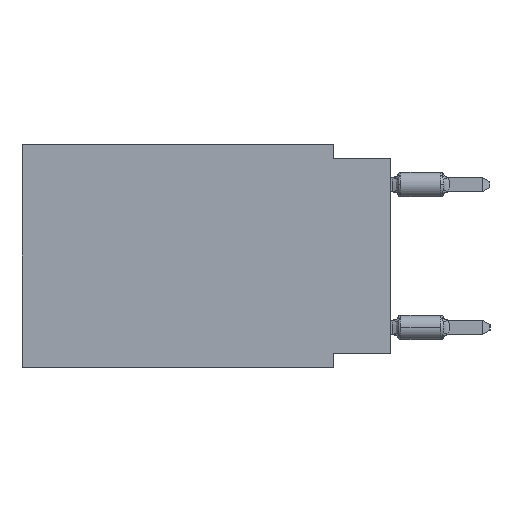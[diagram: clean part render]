
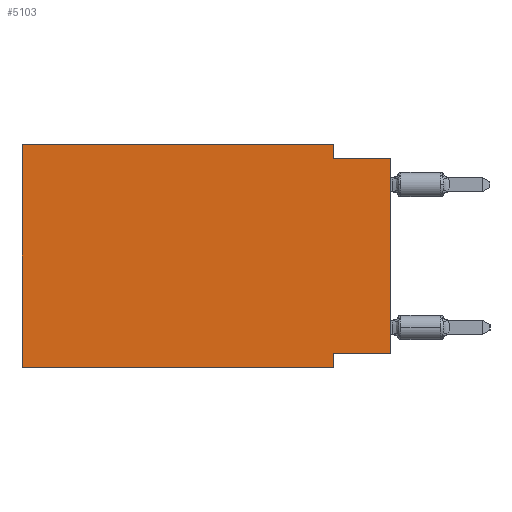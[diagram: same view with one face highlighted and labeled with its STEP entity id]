
A CAD part, left-side view. The second image highlights one B-rep face of the part: STEP entity #5103.
In plain terms, the highlighted planar face has unit normal (-1, 0, 0).
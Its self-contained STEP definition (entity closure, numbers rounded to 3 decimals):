
#9 = DIRECTION ( 'NONE',  ( 0., -1., 0. ) ) ;
#330 = CARTESIAN_POINT ( 'NONE',  ( 0., 0., -9.271 ) ) ;
#332 = EDGE_LOOP ( 'NONE', ( #17485, #18186, #5231, #24976, #13403, #13061, #11754, #11961 ) ) ;
#1026 = VECTOR ( 'NONE', #8580, 1000. ) ;
#1170 = DIRECTION ( 'NONE',  ( 0., 0., -1. ) ) ;
#1179 = VECTOR ( 'NONE', #9, 1000. ) ;
#2047 = VECTOR ( 'NONE', #16837, 1000. ) ;
#2448 = AXIS2_PLACEMENT_3D ( 'NONE', #17771, #19978, #12209 ) ;
#3163 = CARTESIAN_POINT ( 'NONE',  ( 0., 0., -0.635 ) ) ;
#3416 = CARTESIAN_POINT ( 'NONE',  ( 0., 16.383, -9.906 ) ) ;
#3505 = CARTESIAN_POINT ( 'NONE',  ( 0., 2.54, -9.906 ) ) ;
#3660 = LINE ( 'NONE', #21502, #12618 ) ;
#3686 = EDGE_CURVE ( 'NONE', #25489, #17269, #23426, .T. ) ;
#4544 = CARTESIAN_POINT ( 'NONE',  ( 0., 2.54, -9.271 ) ) ;
#4808 = LINE ( 'NONE', #330, #2047 ) ;
#5103 = ADVANCED_FACE ( 'NONE', ( #13883 ), #6258, .F. ) ;
#5215 = VECTOR ( 'NONE', #1170, 1000. ) ;
#5231 = ORIENTED_EDGE ( 'NONE', *, *, #6964, .F. ) ;
#5318 = LINE ( 'NONE', #10995, #18432 ) ;
#6258 = PLANE ( 'NONE',  #2448 ) ;
#6593 = DIRECTION ( 'NONE',  ( 0., 0., 1. ) ) ;
#6964 = EDGE_CURVE ( 'NONE', #10859, #25489, #16692, .T. ) ;
#7289 = LINE ( 'NONE', #3416, #22539 ) ;
#8030 = CARTESIAN_POINT ( 'NONE',  ( 0., 0., -0.635 ) ) ;
#8580 = DIRECTION ( 'NONE',  ( 0., -1., 0. ) ) ;
#9978 = VERTEX_POINT ( 'NONE', #3505 ) ;
#9992 = VERTEX_POINT ( 'NONE', #11254 ) ;
#10859 = VERTEX_POINT ( 'NONE', #16098 ) ;
#10995 = CARTESIAN_POINT ( 'NONE',  ( 0., 2.54, -9.906 ) ) ;
#11254 = CARTESIAN_POINT ( 'NONE',  ( 0., 0., -9.271 ) ) ;
#11754 = ORIENTED_EDGE ( 'NONE', *, *, #22103, .F. ) ;
#11961 = ORIENTED_EDGE ( 'NONE', *, *, #18721, .F. ) ;
#12209 = DIRECTION ( 'NONE',  ( 0., 0., -1. ) ) ;
#12470 = LINE ( 'NONE', #16864, #1026 ) ;
#12567 = VERTEX_POINT ( 'NONE', #4544 ) ;
#12618 = VECTOR ( 'NONE', #17362, 1000. ) ;
#13061 = ORIENTED_EDGE ( 'NONE', *, *, #23484, .T. ) ;
#13403 = ORIENTED_EDGE ( 'NONE', *, *, #19513, .F. ) ;
#13804 = VERTEX_POINT ( 'NONE', #15860 ) ;
#13883 = FACE_OUTER_BOUND ( 'NONE', #332, .T. ) ;
#14854 = LINE ( 'NONE', #24436, #19285 ) ;
#15860 = CARTESIAN_POINT ( 'NONE',  ( 0., 16.383, -9.906 ) ) ;
#16098 = CARTESIAN_POINT ( 'NONE',  ( 0., 2.54, 0. ) ) ;
#16692 = LINE ( 'NONE', #16948, #5215 ) ;
#16837 = DIRECTION ( 'NONE',  ( 0., 1., 0. ) ) ;
#16864 = CARTESIAN_POINT ( 'NONE',  ( 0., 16.383, 0. ) ) ;
#16948 = CARTESIAN_POINT ( 'NONE',  ( 0., 2.54, 0. ) ) ;
#17250 = EDGE_CURVE ( 'NONE', #20992, #10859, #12470, .T. ) ;
#17269 = VERTEX_POINT ( 'NONE', #3163 ) ;
#17362 = DIRECTION ( 'NONE',  ( 0., 0., 1. ) ) ;
#17443 = EDGE_CURVE ( 'NONE', #9992, #17269, #3660, .T. ) ;
#17485 = ORIENTED_EDGE ( 'NONE', *, *, #17443, .T. ) ;
#17771 = CARTESIAN_POINT ( 'NONE',  ( 0., 16.383, 0. ) ) ;
#18186 = ORIENTED_EDGE ( 'NONE', *, *, #3686, .F. ) ;
#18432 = VECTOR ( 'NONE', #18771, 1000. ) ;
#18721 = EDGE_CURVE ( 'NONE', #9992, #12567, #4808, .T. ) ;
#18771 = DIRECTION ( 'NONE',  ( 0., 0., -1. ) ) ;
#19285 = VECTOR ( 'NONE', #6593, 1000. ) ;
#19513 = EDGE_CURVE ( 'NONE', #13804, #20992, #14854, .T. ) ;
#19978 = DIRECTION ( 'NONE',  ( 1., 0., 0. ) ) ;
#20992 = VERTEX_POINT ( 'NONE', #25355 ) ;
#21502 = CARTESIAN_POINT ( 'NONE',  ( 0., 0., 0. ) ) ;
#22103 = EDGE_CURVE ( 'NONE', #12567, #9978, #5318, .T. ) ;
#22539 = VECTOR ( 'NONE', #23067, 1000. ) ;
#23067 = DIRECTION ( 'NONE',  ( 0., -1., 0. ) ) ;
#23426 = LINE ( 'NONE', #8030, #1179 ) ;
#23484 = EDGE_CURVE ( 'NONE', #13804, #9978, #7289, .T. ) ;
#24436 = CARTESIAN_POINT ( 'NONE',  ( 0., 16.383, 0. ) ) ;
#24829 = CARTESIAN_POINT ( 'NONE',  ( 0., 2.54, -0.635 ) ) ;
#24976 = ORIENTED_EDGE ( 'NONE', *, *, #17250, .F. ) ;
#25355 = CARTESIAN_POINT ( 'NONE',  ( 0., 16.383, 0. ) ) ;
#25489 = VERTEX_POINT ( 'NONE', #24829 ) ;
